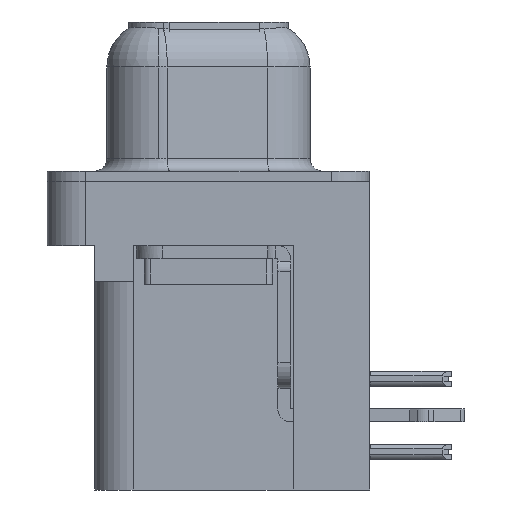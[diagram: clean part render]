
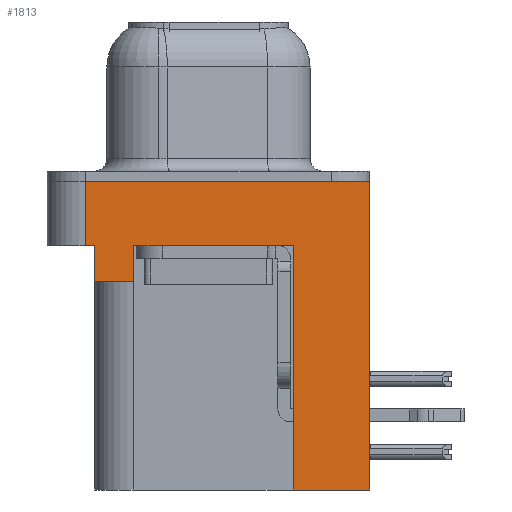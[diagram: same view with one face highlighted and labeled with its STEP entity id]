
A CAD part, left-side view. The second image highlights one B-rep face of the part: STEP entity #1813.
In plain terms, the highlighted planar face has unit normal (-1, 0, 0).
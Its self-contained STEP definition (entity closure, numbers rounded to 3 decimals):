
#697 = EDGE_CURVE ( 'NONE', #14554, #3160, #19158, .T. ) ;
#1146 = AXIS2_PLACEMENT_3D ( 'NONE', #22693, #1471, #26775 ) ;
#1376 = PLANE ( 'NONE',  #1146 ) ;
#1380 = VECTOR ( 'NONE', #3151, 1000. ) ;
#1471 = DIRECTION ( 'NONE',  ( -1., 0., 0. ) ) ;
#1675 = VECTOR ( 'NONE', #25439, 1000. ) ;
#1813 = ADVANCED_FACE ( 'NONE', ( #15195 ), #1376, .T. ) ;
#2241 = VECTOR ( 'NONE', #22861, 1000. ) ;
#2349 = EDGE_CURVE ( 'NONE', #23868, #24859, #12493, .T. ) ;
#3151 = DIRECTION ( 'NONE',  ( 0., 0., 1. ) ) ;
#3160 = VERTEX_POINT ( 'NONE', #17819 ) ;
#3259 = LINE ( 'NONE', #22567, #23882 ) ;
#3320 = VECTOR ( 'NONE', #6620, 1000. ) ;
#3798 = CARTESIAN_POINT ( 'NONE',  ( -2.935, -6.275, -2.5 ) ) ;
#3954 = ORIENTED_EDGE ( 'NONE', *, *, #26271, .T. ) ;
#4045 = CARTESIAN_POINT ( 'NONE',  ( -2.935, -3.295, -2.5 ) ) ;
#4056 = CARTESIAN_POINT ( 'NONE',  ( -2.935, -3.295, -12. ) ) ;
#4108 = EDGE_CURVE ( 'NONE', #18292, #22336, #3259, .T. ) ;
#5484 = VECTOR ( 'NONE', #9884, 1000. ) ;
#5726 = EDGE_CURVE ( 'NONE', #3160, #16359, #10325, .T. ) ;
#6472 = CARTESIAN_POINT ( 'NONE',  ( -2.935, 4.425, -2.5 ) ) ;
#6620 = DIRECTION ( 'NONE',  ( 0., 0., 1. ) ) ;
#7100 = CARTESIAN_POINT ( 'NONE',  ( -2.935, 2.895, -2.5 ) ) ;
#7782 = CARTESIAN_POINT ( 'NONE',  ( -2.935, -6.275, -2.5 ) ) ;
#7806 = LINE ( 'NONE', #3798, #2241 ) ;
#8381 = ORIENTED_EDGE ( 'NONE', *, *, #4108, .F. ) ;
#8700 = EDGE_LOOP ( 'NONE', ( #8381, #9837, #19965, #23684, #17743, #19754, #17981, #13395, #25611, #3954 ) ) ;
#8869 = LINE ( 'NONE', #22876, #3320 ) ;
#8927 = CARTESIAN_POINT ( 'NONE',  ( -2.935, -3.295, -12. ) ) ;
#9269 = EDGE_CURVE ( 'NONE', #10987, #23868, #10344, .T. ) ;
#9674 = VECTOR ( 'NONE', #16733, 1000. ) ;
#9837 = ORIENTED_EDGE ( 'NONE', *, *, #22554, .F. ) ;
#9884 = DIRECTION ( 'NONE',  ( 0., 0., 1. ) ) ;
#9897 = CARTESIAN_POINT ( 'NONE',  ( -2.935, 4.425, -3.9 ) ) ;
#10325 = LINE ( 'NONE', #9897, #24810 ) ;
#10344 = LINE ( 'NONE', #4056, #9674 ) ;
#10987 = VERTEX_POINT ( 'NONE', #25971 ) ;
#11166 = LINE ( 'NONE', #27233, #13508 ) ;
#11495 = DIRECTION ( 'NONE',  ( 0., 1., 0. ) ) ;
#11506 = CARTESIAN_POINT ( 'NONE',  ( -2.935, -3.295, -12. ) ) ;
#12493 = LINE ( 'NONE', #11506, #1675 ) ;
#12562 = LINE ( 'NONE', #13215, #1380 ) ;
#13215 = CARTESIAN_POINT ( 'NONE',  ( -2.935, 4.775, -2.5 ) ) ;
#13395 = ORIENTED_EDGE ( 'NONE', *, *, #2349, .F. ) ;
#13508 = VECTOR ( 'NONE', #16741, 1000. ) ;
#14554 = VERTEX_POINT ( 'NONE', #16804 ) ;
#15195 = FACE_OUTER_BOUND ( 'NONE', #8700, .T. ) ;
#15863 = CARTESIAN_POINT ( 'NONE',  ( -2.935, 4.425, -3.9 ) ) ;
#16359 = VERTEX_POINT ( 'NONE', #6472 ) ;
#16733 = DIRECTION ( 'NONE',  ( 0., 1., 0. ) ) ;
#16741 = DIRECTION ( 'NONE',  ( 0., -1., 0. ) ) ;
#16804 = CARTESIAN_POINT ( 'NONE',  ( -2.935, 2.895, -3.9 ) ) ;
#16946 = EDGE_CURVE ( 'NONE', #14554, #21629, #8869, .T. ) ;
#17743 = ORIENTED_EDGE ( 'NONE', *, *, #697, .F. ) ;
#17778 = CARTESIAN_POINT ( 'NONE',  ( -2.935, -6.275, 0. ) ) ;
#17819 = CARTESIAN_POINT ( 'NONE',  ( -2.935, 4.425, -3.9 ) ) ;
#17981 = ORIENTED_EDGE ( 'NONE', *, *, #18655, .T. ) ;
#18292 = VERTEX_POINT ( 'NONE', #20580 ) ;
#18366 = DIRECTION ( 'NONE',  ( 0., 0., 1. ) ) ;
#18655 = EDGE_CURVE ( 'NONE', #21629, #24859, #7806, .T. ) ;
#19158 = LINE ( 'NONE', #15863, #26087 ) ;
#19310 = VERTEX_POINT ( 'NONE', #19860 ) ;
#19754 = ORIENTED_EDGE ( 'NONE', *, *, #16946, .T. ) ;
#19860 = CARTESIAN_POINT ( 'NONE',  ( -2.935, 4.775, -2.5 ) ) ;
#19965 = ORIENTED_EDGE ( 'NONE', *, *, #23070, .T. ) ;
#20425 = DIRECTION ( 'NONE',  ( 0., -1., 0. ) ) ;
#20580 = CARTESIAN_POINT ( 'NONE',  ( -2.935, 4.775, 0. ) ) ;
#21629 = VERTEX_POINT ( 'NONE', #7100 ) ;
#22336 = VERTEX_POINT ( 'NONE', #17778 ) ;
#22554 = EDGE_CURVE ( 'NONE', #19310, #18292, #12562, .T. ) ;
#22567 = CARTESIAN_POINT ( 'NONE',  ( -2.935, -6.275, 0. ) ) ;
#22693 = CARTESIAN_POINT ( 'NONE',  ( -2.935, -6.275, -2.5 ) ) ;
#22861 = DIRECTION ( 'NONE',  ( 0., -1., 0. ) ) ;
#22876 = CARTESIAN_POINT ( 'NONE',  ( -2.935, 2.895, -3.9 ) ) ;
#23070 = EDGE_CURVE ( 'NONE', #19310, #16359, #11166, .T. ) ;
#23684 = ORIENTED_EDGE ( 'NONE', *, *, #5726, .F. ) ;
#23868 = VERTEX_POINT ( 'NONE', #8927 ) ;
#23882 = VECTOR ( 'NONE', #20425, 1000. ) ;
#24522 = LINE ( 'NONE', #7782, #5484 ) ;
#24810 = VECTOR ( 'NONE', #18366, 1000. ) ;
#24859 = VERTEX_POINT ( 'NONE', #4045 ) ;
#25439 = DIRECTION ( 'NONE',  ( 0., 0., 1. ) ) ;
#25611 = ORIENTED_EDGE ( 'NONE', *, *, #9269, .F. ) ;
#25971 = CARTESIAN_POINT ( 'NONE',  ( -2.935, -6.275, -12. ) ) ;
#26087 = VECTOR ( 'NONE', #11495, 1000. ) ;
#26271 = EDGE_CURVE ( 'NONE', #10987, #22336, #24522, .T. ) ;
#26775 = DIRECTION ( 'NONE',  ( 0., 0., 1. ) ) ;
#27233 = CARTESIAN_POINT ( 'NONE',  ( -2.935, -6.275, -2.5 ) ) ;
